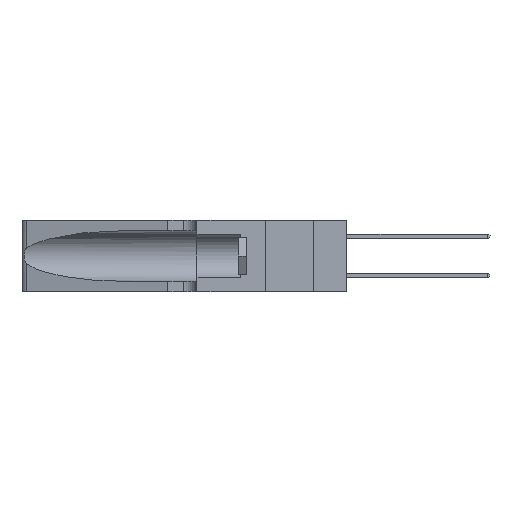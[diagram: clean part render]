
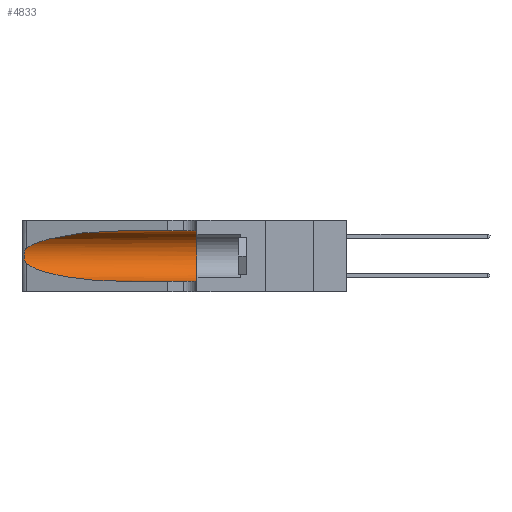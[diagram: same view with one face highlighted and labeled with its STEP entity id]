
A CAD part, left-side view. The second image highlights one B-rep face of the part: STEP entity #4833.
In plain terms, the highlighted cylindrical face has radius 3.308 mm (diameter 6.617 mm), a partial arc.
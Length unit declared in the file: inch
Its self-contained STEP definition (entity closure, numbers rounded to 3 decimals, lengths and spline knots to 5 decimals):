
#494 = AXIS2_PLACEMENT_3D ( 'NONE', #22564, #5650, #7801 ) ;
#1700 = CARTESIAN_POINT ( 'NONE',  ( 0.18966, 0.96281, 0.05475 ) ) ;
#2068 = ORIENTED_EDGE ( 'NONE', *, *, #26688, .T. ) ;
#3036 = CARTESIAN_POINT ( 'NONE',  ( 0.1305, 1.61858, 0.05475 ) ) ;
#3186 = VERTEX_POINT ( 'NONE', #8954 ) ;
#3421 = CARTESIAN_POINT ( 'NONE',  ( 0.1305, 0.72297, 0.31525 ) ) ;
#3546 = CARTESIAN_POINT ( 'NONE',  ( 0.25487, 1.22718, 0.22369 ) ) ;
#3757 = ORIENTED_EDGE ( 'NONE', *, *, #21409, .T. ) ;
#4833 = ADVANCED_FACE ( 'NONE', ( #27909 ), #21425, .F. ) ;
#5237 = CARTESIAN_POINT ( 'NONE',  ( 0.25555, 1.22993, 0.14849 ) ) ;
#5650 = DIRECTION ( 'NONE',  ( 0., -1., 0. ) ) ;
#6414 = CARTESIAN_POINT ( 'NONE',  ( 0.25487, 1.22718, 0.14631 ) ) ;
#7706 = CARTESIAN_POINT ( 'NONE',  ( 0.25487, 1.22718, 0.14631 ) ) ;
#7801 = DIRECTION ( 'NONE',  ( 0., 0., -1. ) ) ;
#8800 = VERTEX_POINT ( 'NONE', #25781 ) ;
#8954 = CARTESIAN_POINT ( 'NONE',  ( 0.25487, 1.22718, 0.14631 ) ) ;
#9558 = LINE ( 'NONE', #3036, #26094 ) ;
#9887 = LINE ( 'NONE', #19383, #12525 ) ;
#9985 = CARTESIAN_POINT ( 'NONE',  ( 0.26017, 1.23833, 0.17102 ) ) ;
#10866 = CARTESIAN_POINT ( 'NONE',  ( 0.1305, 0.72297, 0.05475 ) ) ;
#11758 = VERTEX_POINT ( 'NONE', #10866 ) ;
#12333 = VERTEX_POINT ( 'NONE', #3546 ) ;
#12420 = CARTESIAN_POINT ( 'NONE',  ( 0.25789, 1.23486, 0.15765 ) ) ;
#12525 = VECTOR ( 'NONE', #31621, 39.37008 ) ;
#12986 = EDGE_CURVE ( 'NONE', #8800, #13842, #16405, .T. ) ;
#13384 = ORIENTED_EDGE ( 'NONE', *, *, #22895, .T. ) ;
#13842 = VERTEX_POINT ( 'NONE', #15887 ) ;
#13918 = CARTESIAN_POINT ( 'NONE',  ( 0.2373, 1.15595, 0.08982 ) ) ;
#14146 = VERTEX_POINT ( 'NONE', #18566 ) ;
#14519 =( BOUNDED_CURVE ( )  B_SPLINE_CURVE ( 3, ( #3421, #25920, #15676, #28271 ),
 .UNSPECIFIED., .F., .F. ) 
 B_SPLINE_CURVE_WITH_KNOTS ( ( 4, 4 ),
 ( 1.5708, 2.84003 ),
 .UNSPECIFIED. ) 
 CURVE ( )  GEOMETRIC_REPRESENTATION_ITEM ( )  RATIONAL_B_SPLINE_CURVE ( ( 1., 0.87, 0.87, 1. ) ) 
 REPRESENTATION_ITEM ( '' )  );
#14803 = CARTESIAN_POINT ( 'NONE',  ( 0.26018, 1.23835, 0.19895 ) ) ;
#14977 = DIRECTION ( 'NONE',  ( 0., -1., 0. ) ) ;
#15676 = CARTESIAN_POINT ( 'NONE',  ( 0.2373, 1.15595, 0.28018 ) ) ;
#15887 = CARTESIAN_POINT ( 'NONE',  ( 0.1305, 0.35, 0.05475 ) ) ;
#15958 = ORIENTED_EDGE ( 'NONE', *, *, #30137, .F. ) ;
#16405 = CIRCLE ( 'NONE', #23167, 0.13025 ) ;
#17486 = CARTESIAN_POINT ( 'NONE',  ( 0.25854, 1.2359, 0.20912 ) ) ;
#18566 = CARTESIAN_POINT ( 'NONE',  ( 0.1305, 0.72297, 0.31525 ) ) ;
#19383 = CARTESIAN_POINT ( 'NONE',  ( 0.1305, 1.61858, 0.31525 ) ) ;
#19420 = EDGE_LOOP ( 'NONE', ( #3757, #20112, #13384, #2068, #23289, #15958 ) ) ;
#19986 = CARTESIAN_POINT ( 'NONE',  ( 0.25639, 1.23186, 0.15144 ) ) ;
#20084 = CARTESIAN_POINT ( 'NONE',  ( 0.26075, 1.23896, 0.178 ) ) ;
#20112 = ORIENTED_EDGE ( 'NONE', *, *, #27932, .T. ) ;
#21409 = EDGE_CURVE ( 'NONE', #14146, #12333, #14519, .T. ) ;
#21425 = CYLINDRICAL_SURFACE ( 'NONE', #494, 0.13025 ) ;
#21670 = B_SPLINE_CURVE_WITH_KNOTS ( 'NONE', 3,
 ( #29756, #24827, #29664, #22161, #17486, #14803, #24730, #20084, #9985, #27190, #12420, #19986, #5237, #7706 ),
 .UNSPECIFIED., .F., .F.,
 ( 4, 2, 2, 2, 2, 2, 4 ),
 ( 0., 0.00027, 0.00053, 0.00107, 0.0016, 0.00187, 0.00214 ),
 .UNSPECIFIED. ) ;
#22161 = CARTESIAN_POINT ( 'NONE',  ( 0.25787, 1.23484, 0.2124 ) ) ;
#22564 = CARTESIAN_POINT ( 'NONE',  ( 0.1305, 1.61858, 0.185 ) ) ;
#22607 =( BOUNDED_CURVE ( )  B_SPLINE_CURVE ( 3, ( #6414, #13918, #1700, #23853 ),
 .UNSPECIFIED., .F., .F. ) 
 B_SPLINE_CURVE_WITH_KNOTS ( ( 4, 4 ),
 ( 3.44316, 4.71239 ),
 .UNSPECIFIED. ) 
 CURVE ( )  GEOMETRIC_REPRESENTATION_ITEM ( )  RATIONAL_B_SPLINE_CURVE ( ( 1., 0.87, 0.87, 1. ) ) 
 REPRESENTATION_ITEM ( '' )  );
#22895 = EDGE_CURVE ( 'NONE', #3186, #11758, #22607, .T. ) ;
#23157 = DIRECTION ( 'NONE',  ( 0., 1., 0. ) ) ;
#23167 = AXIS2_PLACEMENT_3D ( 'NONE', #25868, #23157, #27995 ) ;
#23289 = ORIENTED_EDGE ( 'NONE', *, *, #12986, .F. ) ;
#23853 = CARTESIAN_POINT ( 'NONE',  ( 0.1305, 0.72297, 0.05475 ) ) ;
#24730 = CARTESIAN_POINT ( 'NONE',  ( 0.26075, 1.23896, 0.19203 ) ) ;
#24827 = CARTESIAN_POINT ( 'NONE',  ( 0.25555, 1.22994, 0.2215 ) ) ;
#25781 = CARTESIAN_POINT ( 'NONE',  ( 0.1305, 0.35, 0.31525 ) ) ;
#25868 = CARTESIAN_POINT ( 'NONE',  ( 0.1305, 0.35, 0.185 ) ) ;
#25920 = CARTESIAN_POINT ( 'NONE',  ( 0.18966, 0.96281, 0.31525 ) ) ;
#26094 = VECTOR ( 'NONE', #14977, 39.37008 ) ;
#26688 = EDGE_CURVE ( 'NONE', #11758, #13842, #9558, .T. ) ;
#27190 = CARTESIAN_POINT ( 'NONE',  ( 0.25856, 1.23593, 0.16098 ) ) ;
#27909 = FACE_OUTER_BOUND ( 'NONE', #19420, .T. ) ;
#27932 = EDGE_CURVE ( 'NONE', #12333, #3186, #21670, .T. ) ;
#27995 = DIRECTION ( 'NONE',  ( 0., 0., 1. ) ) ;
#28271 = CARTESIAN_POINT ( 'NONE',  ( 0.25487, 1.22718, 0.22369 ) ) ;
#29664 = CARTESIAN_POINT ( 'NONE',  ( 0.25639, 1.23184, 0.21858 ) ) ;
#29756 = CARTESIAN_POINT ( 'NONE',  ( 0.25487, 1.22718, 0.22369 ) ) ;
#30137 = EDGE_CURVE ( 'NONE', #14146, #8800, #9887, .T. ) ;
#31621 = DIRECTION ( 'NONE',  ( 0., -1., 0. ) ) ;
